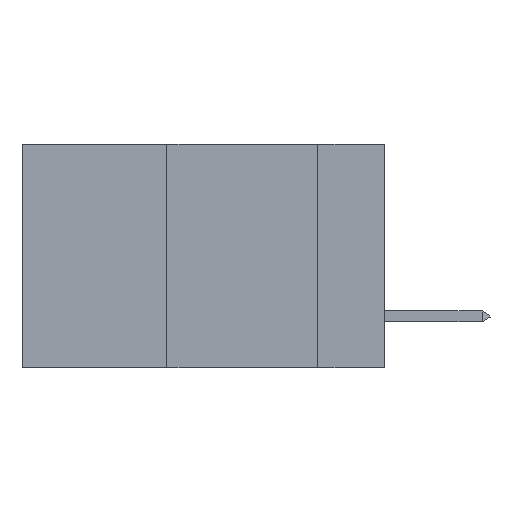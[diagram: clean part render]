
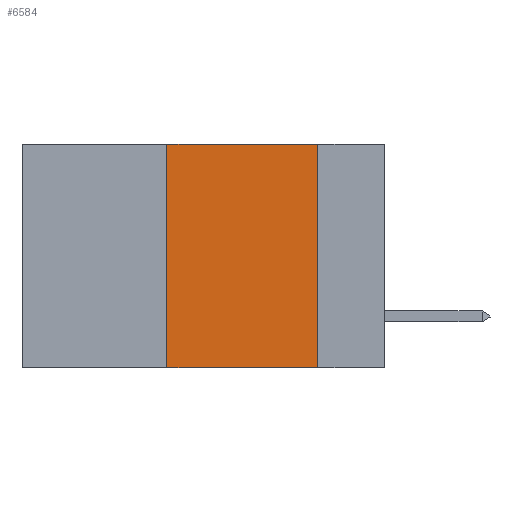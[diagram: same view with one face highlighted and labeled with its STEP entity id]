
A CAD part, left-side view. The second image highlights one B-rep face of the part: STEP entity #6584.
In plain terms, the highlighted planar face has unit normal (-1, 0, 0).
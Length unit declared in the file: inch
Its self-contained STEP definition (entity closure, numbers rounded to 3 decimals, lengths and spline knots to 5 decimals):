
#274 = VECTOR ( 'NONE', #19908, 39.37008 ) ;
#950 = VERTEX_POINT ( 'NONE', #16862 ) ;
#956 = ORIENTED_EDGE ( 'NONE', *, *, #11005, .F. ) ;
#1074 = LINE ( 'NONE', #18940, #10118 ) ;
#1383 = FACE_OUTER_BOUND ( 'NONE', #22267, .T. ) ;
#2093 = CARTESIAN_POINT ( 'NONE',  ( 0., 0.6, 0. ) ) ;
#2669 = ORIENTED_EDGE ( 'NONE', *, *, #5024, .F. ) ;
#3084 = PLANE ( 'NONE',  #11614 ) ;
#3538 = VERTEX_POINT ( 'NONE', #3587 ) ;
#3587 = CARTESIAN_POINT ( 'NONE',  ( 0., 0.11, -0.37 ) ) ;
#3664 = EDGE_CURVE ( 'NONE', #14419, #3538, #5706, .T. ) ;
#4760 = DIRECTION ( 'NONE',  ( 0., -1., 0. ) ) ;
#4888 = DIRECTION ( 'NONE',  ( 0., 0., -1. ) ) ;
#5024 = EDGE_CURVE ( 'NONE', #950, #13196, #9852, .T. ) ;
#5063 = VECTOR ( 'NONE', #21953, 39.37008 ) ;
#5137 = VECTOR ( 'NONE', #11211, 39.37008 ) ;
#5209 = CARTESIAN_POINT ( 'NONE',  ( 0., 0.11, 0. ) ) ;
#5216 = EDGE_CURVE ( 'NONE', #950, #3538, #1074, .T. ) ;
#5706 = LINE ( 'NONE', #7592, #5137 ) ;
#6584 = ADVANCED_FACE ( 'NONE', ( #1383 ), #3084, .F. ) ;
#7592 = CARTESIAN_POINT ( 'NONE',  ( 0., 0.11, 0. ) ) ;
#9852 = LINE ( 'NONE', #16652, #5063 ) ;
#9911 = LINE ( 'NONE', #2093, #274 ) ;
#10118 = VECTOR ( 'NONE', #4760, 39.37008 ) ;
#10281 = ORIENTED_EDGE ( 'NONE', *, *, #5216, .T. ) ;
#11005 = EDGE_CURVE ( 'NONE', #13196, #14419, #9911, .T. ) ;
#11211 = DIRECTION ( 'NONE',  ( 0., 0., -1. ) ) ;
#11614 = AXIS2_PLACEMENT_3D ( 'NONE', #20836, #15599, #4888 ) ;
#12681 = ORIENTED_EDGE ( 'NONE', *, *, #3664, .F. ) ;
#13196 = VERTEX_POINT ( 'NONE', #17513 ) ;
#14419 = VERTEX_POINT ( 'NONE', #5209 ) ;
#15599 = DIRECTION ( 'NONE',  ( 1., 0., 0. ) ) ;
#16652 = CARTESIAN_POINT ( 'NONE',  ( 0., 0.36, 0. ) ) ;
#16862 = CARTESIAN_POINT ( 'NONE',  ( 0., 0.36, -0.37 ) ) ;
#17513 = CARTESIAN_POINT ( 'NONE',  ( 0., 0.36, 0. ) ) ;
#18940 = CARTESIAN_POINT ( 'NONE',  ( 0., 0.6, -0.37 ) ) ;
#19908 = DIRECTION ( 'NONE',  ( 0., -1., 0. ) ) ;
#20836 = CARTESIAN_POINT ( 'NONE',  ( 0., 0.6, 0. ) ) ;
#21953 = DIRECTION ( 'NONE',  ( 0., 0., 1. ) ) ;
#22267 = EDGE_LOOP ( 'NONE', ( #12681, #956, #2669, #10281 ) ) ;
